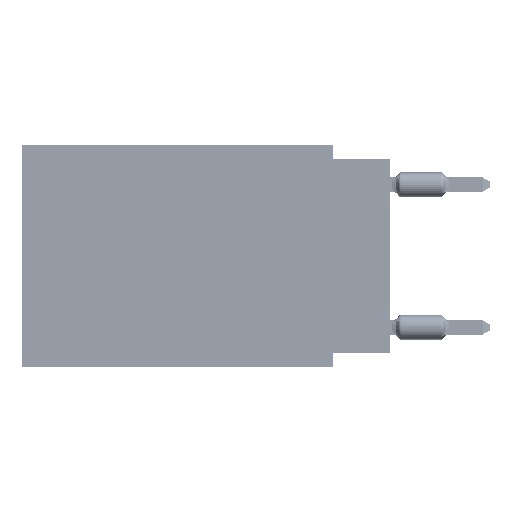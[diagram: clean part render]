
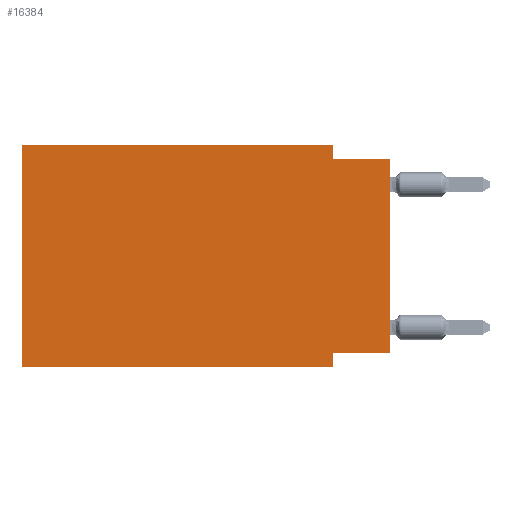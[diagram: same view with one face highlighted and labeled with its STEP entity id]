
A CAD part, left-side view. The second image highlights one B-rep face of the part: STEP entity #16384.
In plain terms, the highlighted planar face has unit normal (-1, 0, 0).
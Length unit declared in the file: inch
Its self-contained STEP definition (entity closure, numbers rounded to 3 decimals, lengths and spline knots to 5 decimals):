
#937 = FACE_OUTER_BOUND ( 'NONE', #23296, .T. ) ;
#2445 = CARTESIAN_POINT ( 'NONE',  ( 0., 0.645, 0. ) ) ;
#7351 = VERTEX_POINT ( 'NONE', #25064 ) ;
#8111 = LINE ( 'NONE', #61953, #47682 ) ;
#8426 = DIRECTION ( 'NONE',  ( 0., -1., 0. ) ) ;
#9524 = CARTESIAN_POINT ( 'NONE',  ( 0., 0.645, -0.39 ) ) ;
#11068 = CARTESIAN_POINT ( 'NONE',  ( 0., 0.645, 0. ) ) ;
#11586 = DIRECTION ( 'NONE',  ( 0., 1., 0. ) ) ;
#12368 = LINE ( 'NONE', #40624, #35796 ) ;
#13050 = CARTESIAN_POINT ( 'NONE',  ( 0., 0., -0.365 ) ) ;
#15043 = CARTESIAN_POINT ( 'NONE',  ( 0., 0., -0.025 ) ) ;
#15691 = AXIS2_PLACEMENT_3D ( 'NONE', #47746, #80840, #74644 ) ;
#16384 = ADVANCED_FACE ( 'NONE', ( #937 ), #53916, .F. ) ;
#17994 = VERTEX_POINT ( 'NONE', #28211 ) ;
#22931 = CARTESIAN_POINT ( 'NONE',  ( 0., 0.1, -0.365 ) ) ;
#23296 = EDGE_LOOP ( 'NONE', ( #44801, #38212, #86642, #58726, #86857, #41869, #34342, #30705 ) ) ;
#23647 = CARTESIAN_POINT ( 'NONE',  ( 0., 0.1, -0.39 ) ) ;
#25064 = CARTESIAN_POINT ( 'NONE',  ( 0., 0.1, -0.025 ) ) ;
#26146 = CARTESIAN_POINT ( 'NONE',  ( 0., 0., -0.365 ) ) ;
#28211 = CARTESIAN_POINT ( 'NONE',  ( 0., 0.1, 0. ) ) ;
#29288 = VECTOR ( 'NONE', #49288, 39.37008 ) ;
#30705 = ORIENTED_EDGE ( 'NONE', *, *, #36101, .F. ) ;
#31622 = VERTEX_POINT ( 'NONE', #85680 ) ;
#34342 = ORIENTED_EDGE ( 'NONE', *, *, #49909, .F. ) ;
#35796 = VECTOR ( 'NONE', #60456, 39.37008 ) ;
#36101 = EDGE_CURVE ( 'NONE', #42788, #56632, #79997, .T. ) ;
#36896 = CARTESIAN_POINT ( 'NONE',  ( 0., 0.1, -0.39 ) ) ;
#38212 = ORIENTED_EDGE ( 'NONE', *, *, #82036, .F. ) ;
#40435 = EDGE_CURVE ( 'NONE', #67451, #31622, #78158, .T. ) ;
#40624 = CARTESIAN_POINT ( 'NONE',  ( 0., 0., 0. ) ) ;
#41869 = ORIENTED_EDGE ( 'NONE', *, *, #60851, .T. ) ;
#42788 = VERTEX_POINT ( 'NONE', #13050 ) ;
#44801 = ORIENTED_EDGE ( 'NONE', *, *, #45152, .T. ) ;
#45152 = EDGE_CURVE ( 'NONE', #42788, #68544, #12368, .T. ) ;
#47682 = VECTOR ( 'NONE', #50478, 39.37008 ) ;
#47746 = CARTESIAN_POINT ( 'NONE',  ( 0., 0.645, 0. ) ) ;
#49288 = DIRECTION ( 'NONE',  ( 0., -1., 0. ) ) ;
#49909 = EDGE_CURVE ( 'NONE', #56632, #70433, #57201, .T. ) ;
#50478 = DIRECTION ( 'NONE',  ( 0., 0., -1. ) ) ;
#50543 = DIRECTION ( 'NONE',  ( 0., -1., 0. ) ) ;
#53916 = PLANE ( 'NONE',  #15691 ) ;
#55863 = LINE ( 'NONE', #2445, #79921 ) ;
#56632 = VERTEX_POINT ( 'NONE', #22931 ) ;
#57201 = LINE ( 'NONE', #23647, #67308 ) ;
#58340 = VECTOR ( 'NONE', #11586, 39.37008 ) ;
#58726 = ORIENTED_EDGE ( 'NONE', *, *, #67925, .F. ) ;
#59393 = VECTOR ( 'NONE', #61541, 39.37008 ) ;
#60456 = DIRECTION ( 'NONE',  ( 0., 0., 1. ) ) ;
#60851 = EDGE_CURVE ( 'NONE', #67451, #70433, #74870, .T. ) ;
#61428 = EDGE_CURVE ( 'NONE', #17994, #7351, #8111, .T. ) ;
#61541 = DIRECTION ( 'NONE',  ( 0., 0., 1. ) ) ;
#61953 = CARTESIAN_POINT ( 'NONE',  ( 0., 0.1, 0. ) ) ;
#66154 = CARTESIAN_POINT ( 'NONE',  ( 0., 0., -0.025 ) ) ;
#67308 = VECTOR ( 'NONE', #72157, 39.37008 ) ;
#67413 = CARTESIAN_POINT ( 'NONE',  ( 0., 0.645, -0.39 ) ) ;
#67451 = VERTEX_POINT ( 'NONE', #67413 ) ;
#67925 = EDGE_CURVE ( 'NONE', #31622, #17994, #55863, .T. ) ;
#68544 = VERTEX_POINT ( 'NONE', #66154 ) ;
#69188 = VECTOR ( 'NONE', #8426, 39.37008 ) ;
#70433 = VERTEX_POINT ( 'NONE', #36896 ) ;
#72157 = DIRECTION ( 'NONE',  ( 0., 0., -1. ) ) ;
#74644 = DIRECTION ( 'NONE',  ( 0., 0., -1. ) ) ;
#74870 = LINE ( 'NONE', #9524, #29288 ) ;
#75526 = LINE ( 'NONE', #15043, #69188 ) ;
#78158 = LINE ( 'NONE', #11068, #59393 ) ;
#79921 = VECTOR ( 'NONE', #50543, 39.37008 ) ;
#79997 = LINE ( 'NONE', #26146, #58340 ) ;
#80840 = DIRECTION ( 'NONE',  ( 1., 0., 0. ) ) ;
#82036 = EDGE_CURVE ( 'NONE', #7351, #68544, #75526, .T. ) ;
#85680 = CARTESIAN_POINT ( 'NONE',  ( 0., 0.645, 0. ) ) ;
#86642 = ORIENTED_EDGE ( 'NONE', *, *, #61428, .F. ) ;
#86857 = ORIENTED_EDGE ( 'NONE', *, *, #40435, .F. ) ;
